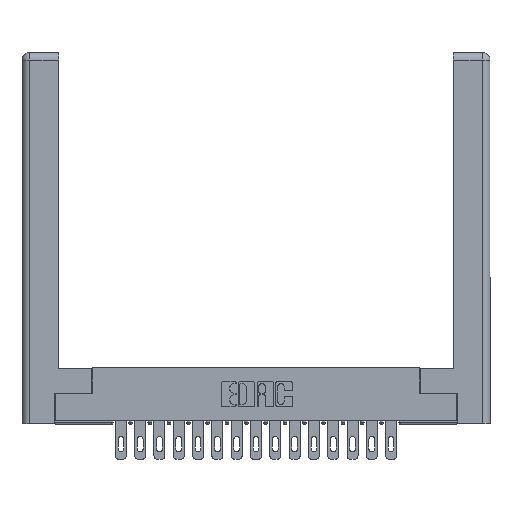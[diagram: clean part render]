
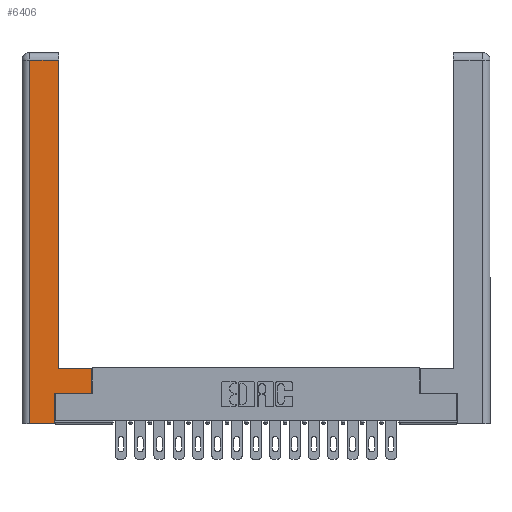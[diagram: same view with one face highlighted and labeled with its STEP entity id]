
A CAD part, top view. The second image highlights one B-rep face of the part: STEP entity #6406.
In plain terms, the highlighted planar face has unit normal (0, 0, 1).
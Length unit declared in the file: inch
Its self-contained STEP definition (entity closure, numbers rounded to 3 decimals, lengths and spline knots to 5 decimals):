
#156 = EDGE_LOOP ( 'NONE', ( #10258, #3786, #10306, #14347, #14025, #708, #12247, #3691 ) ) ;
#382 = EDGE_CURVE ( 'NONE', #13654, #2695, #6295, .T. ) ;
#639 = VERTEX_POINT ( 'NONE', #15621 ) ;
#708 = ORIENTED_EDGE ( 'NONE', *, *, #14959, .T. ) ;
#716 = PLANE ( 'NONE',  #1056 ) ;
#1056 = AXIS2_PLACEMENT_3D ( 'NONE', #12855, #17798, #5984 ) ;
#1980 = VECTOR ( 'NONE', #14172, 39.37008 ) ;
#2695 = VERTEX_POINT ( 'NONE', #15360 ) ;
#2990 = FACE_OUTER_BOUND ( 'NONE', #156, .T. ) ;
#3460 = LINE ( 'NONE', #8639, #16592 ) ;
#3563 = VERTEX_POINT ( 'NONE', #3703 ) ;
#3572 = EDGE_CURVE ( 'NONE', #6640, #3563, #4287, .T. ) ;
#3628 = EDGE_CURVE ( 'NONE', #14644, #8630, #4007, .T. ) ;
#3691 = ORIENTED_EDGE ( 'NONE', *, *, #14794, .T. ) ;
#3703 = CARTESIAN_POINT ( 'NONE',  ( 0.265, 0.245, 0. ) ) ;
#3786 = ORIENTED_EDGE ( 'NONE', *, *, #8633, .T. ) ;
#3850 = DIRECTION ( 'NONE',  ( -1., 0., 0. ) ) ;
#4007 = LINE ( 'NONE', #11071, #9659 ) ;
#4287 = LINE ( 'NONE', #10531, #6199 ) ;
#5984 = DIRECTION ( 'NONE',  ( -1., 0., 0. ) ) ;
#6199 = VECTOR ( 'NONE', #7023, 39.37008 ) ;
#6295 = LINE ( 'NONE', #15185, #21806 ) ;
#6406 = ADVANCED_FACE ( 'NONE', ( #2990 ), #716, .F. ) ;
#6640 = VERTEX_POINT ( 'NONE', #21490 ) ;
#6871 = CARTESIAN_POINT ( 'NONE',  ( 0.265, 0., 0. ) ) ;
#7023 = DIRECTION ( 'NONE',  ( 0., 1., 0. ) ) ;
#7489 = EDGE_CURVE ( 'NONE', #8630, #6640, #8353, .T. ) ;
#7548 = VERTEX_POINT ( 'NONE', #20323 ) ;
#7755 = CARTESIAN_POINT ( 'NONE',  ( 0.295, 0.45, 0. ) ) ;
#8353 = LINE ( 'NONE', #6871, #20942 ) ;
#8630 = VERTEX_POINT ( 'NONE', #14272 ) ;
#8633 = EDGE_CURVE ( 'NONE', #2695, #14644, #17402, .T. ) ;
#8639 = CARTESIAN_POINT ( 'NONE',  ( 0.565, 0.245, 0. ) ) ;
#8930 = CARTESIAN_POINT ( 'NONE',  ( 0.0615, 2.94, 0. ) ) ;
#9377 = LINE ( 'NONE', #12411, #18374 ) ;
#9659 = VECTOR ( 'NONE', #17631, 39.37008 ) ;
#10258 = ORIENTED_EDGE ( 'NONE', *, *, #382, .T. ) ;
#10291 = LINE ( 'NONE', #14460, #1980 ) ;
#10306 = ORIENTED_EDGE ( 'NONE', *, *, #3628, .T. ) ;
#10531 = CARTESIAN_POINT ( 'NONE',  ( 0.265, 0.245, 0. ) ) ;
#11071 = CARTESIAN_POINT ( 'NONE',  ( 0.0615, 0., 0. ) ) ;
#11123 = EDGE_CURVE ( 'NONE', #7548, #639, #10291, .T. ) ;
#11722 = DIRECTION ( 'NONE',  ( 0., 1., 0. ) ) ;
#12247 = ORIENTED_EDGE ( 'NONE', *, *, #11123, .T. ) ;
#12411 = CARTESIAN_POINT ( 'NONE',  ( 0.295, 0.45, 0. ) ) ;
#12720 = CARTESIAN_POINT ( 'NONE',  ( 0.0615, 2.94, 0. ) ) ;
#12855 = CARTESIAN_POINT ( 'NONE',  ( 0., 0., 0. ) ) ;
#13654 = VERTEX_POINT ( 'NONE', #7755 ) ;
#13674 = VECTOR ( 'NONE', #14059, 39.37008 ) ;
#13822 = DIRECTION ( 'NONE',  ( 1., 0., 0. ) ) ;
#14025 = ORIENTED_EDGE ( 'NONE', *, *, #3572, .T. ) ;
#14059 = DIRECTION ( 'NONE',  ( -1., 0., 0. ) ) ;
#14172 = DIRECTION ( 'NONE',  ( 0., 1., 0. ) ) ;
#14272 = CARTESIAN_POINT ( 'NONE',  ( 0.0615, 0., 0. ) ) ;
#14347 = ORIENTED_EDGE ( 'NONE', *, *, #7489, .T. ) ;
#14460 = CARTESIAN_POINT ( 'NONE',  ( 0.565, 0.45, 0. ) ) ;
#14644 = VERTEX_POINT ( 'NONE', #12720 ) ;
#14794 = EDGE_CURVE ( 'NONE', #639, #13654, #9377, .T. ) ;
#14959 = EDGE_CURVE ( 'NONE', #3563, #7548, #3460, .T. ) ;
#15185 = CARTESIAN_POINT ( 'NONE',  ( 0.295, 3., 0. ) ) ;
#15360 = CARTESIAN_POINT ( 'NONE',  ( 0.295, 2.94, 0. ) ) ;
#15488 = DIRECTION ( 'NONE',  ( 1., 0., 0. ) ) ;
#15621 = CARTESIAN_POINT ( 'NONE',  ( 0.565, 0.45, 0. ) ) ;
#16592 = VECTOR ( 'NONE', #13822, 39.37008 ) ;
#17402 = LINE ( 'NONE', #8930, #13674 ) ;
#17631 = DIRECTION ( 'NONE',  ( 0., -1., 0. ) ) ;
#17798 = DIRECTION ( 'NONE',  ( 0., 0., -1. ) ) ;
#18374 = VECTOR ( 'NONE', #3850, 39.37008 ) ;
#20323 = CARTESIAN_POINT ( 'NONE',  ( 0.565, 0.245, 0. ) ) ;
#20942 = VECTOR ( 'NONE', #15488, 39.37008 ) ;
#21490 = CARTESIAN_POINT ( 'NONE',  ( 0.265, 0., 0. ) ) ;
#21806 = VECTOR ( 'NONE', #11722, 39.37008 ) ;
